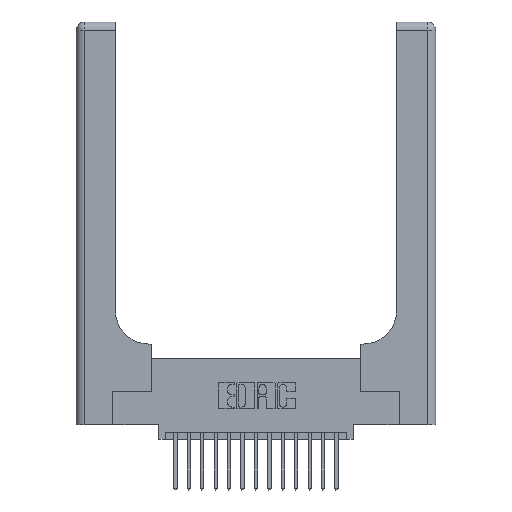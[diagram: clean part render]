
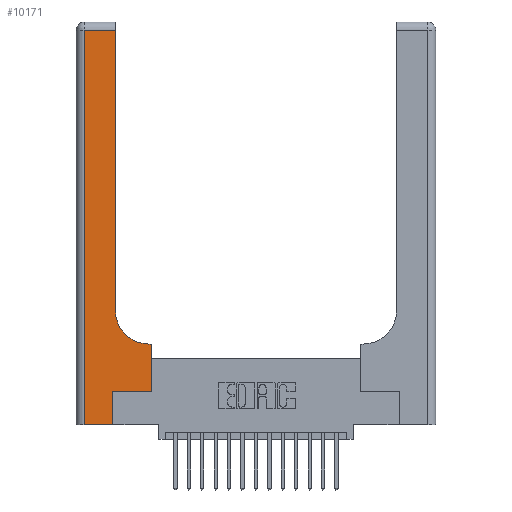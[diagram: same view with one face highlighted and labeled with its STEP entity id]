
A CAD part, top view. The second image highlights one B-rep face of the part: STEP entity #10171.
In plain terms, the highlighted planar face has unit normal (0, 0, 1).
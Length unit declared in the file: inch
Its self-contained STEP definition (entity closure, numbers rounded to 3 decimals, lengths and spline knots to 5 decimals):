
#387 = CARTESIAN_POINT ( 'NONE',  ( 0.5585, 0.25, 0.37 ) ) ;
#643 = VECTOR ( 'NONE', #1100, 39.37008 ) ;
#818 = VECTOR ( 'NONE', #9234, 39.37008 ) ;
#954 = VECTOR ( 'NONE', #3382, 39.37008 ) ;
#1036 = VERTEX_POINT ( 'NONE', #5434 ) ;
#1100 = DIRECTION ( 'NONE',  ( 0., 1., 0. ) ) ;
#1105 = EDGE_CURVE ( 'NONE', #1036, #17673, #13843, .T. ) ;
#1340 = DIRECTION ( 'NONE',  ( 0., 0., -1. ) ) ;
#1770 = CARTESIAN_POINT ( 'NONE',  ( 0., 0., 0.37 ) ) ;
#1915 = CARTESIAN_POINT ( 'NONE',  ( 0.5415, 0.6, 0.37 ) ) ;
#2527 = VECTOR ( 'NONE', #12479, 39.37008 ) ;
#2695 = VERTEX_POINT ( 'NONE', #387 ) ;
#3214 = DIRECTION ( 'NONE',  ( 0., -1., 0. ) ) ;
#3382 = DIRECTION ( 'NONE',  ( 0., 1., 0. ) ) ;
#3685 = ORIENTED_EDGE ( 'NONE', *, *, #6697, .T. ) ;
#3726 = VECTOR ( 'NONE', #6259, 39.37008 ) ;
#3788 = CARTESIAN_POINT ( 'NONE',  ( 0.06, 3., 0.37 ) ) ;
#3835 = VERTEX_POINT ( 'NONE', #15019 ) ;
#3852 = CARTESIAN_POINT ( 'NONE',  ( 0., 3., 0.37 ) ) ;
#5359 = LINE ( 'NONE', #7733, #818 ) ;
#5396 = DIRECTION ( 'NONE',  ( 0., 0., -1. ) ) ;
#5434 = CARTESIAN_POINT ( 'NONE',  ( 0.06, 2.94, 0.37 ) ) ;
#5608 = EDGE_CURVE ( 'NONE', #17673, #18857, #8044, .T. ) ;
#5640 = LINE ( 'NONE', #18066, #16146 ) ;
#5921 = CARTESIAN_POINT ( 'NONE',  ( 0.269, 0., 0.37 ) ) ;
#6138 = ORIENTED_EDGE ( 'NONE', *, *, #1105, .T. ) ;
#6259 = DIRECTION ( 'NONE',  ( 0., 1., 0. ) ) ;
#6562 = LINE ( 'NONE', #18407, #2527 ) ;
#6697 = EDGE_CURVE ( 'NONE', #3835, #1036, #5640, .T. ) ;
#6767 = EDGE_CURVE ( 'NONE', #13712, #3835, #11720, .T. ) ;
#7733 = CARTESIAN_POINT ( 'NONE',  ( 0.2915, 0.6, 0.37 ) ) ;
#7912 = EDGE_CURVE ( 'NONE', #9770, #16740, #5359, .T. ) ;
#8044 = LINE ( 'NONE', #1770, #11524 ) ;
#8713 = LINE ( 'NONE', #19083, #643 ) ;
#8943 = ORIENTED_EDGE ( 'NONE', *, *, #15463, .T. ) ;
#9002 = AXIS2_PLACEMENT_3D ( 'NONE', #10399, #1340, #11905 ) ;
#9234 = DIRECTION ( 'NONE',  ( -1., 0., 0. ) ) ;
#9306 = EDGE_CURVE ( 'NONE', #16740, #13712, #13222, .T. ) ;
#9541 = VERTEX_POINT ( 'NONE', #12407 ) ;
#9770 = VERTEX_POINT ( 'NONE', #17536 ) ;
#10006 = AXIS2_PLACEMENT_3D ( 'NONE', #3852, #5396, #15834 ) ;
#10171 = ADVANCED_FACE ( 'NONE', ( #13188 ), #12836, .F. ) ;
#10252 = ORIENTED_EDGE ( 'NONE', *, *, #9306, .T. ) ;
#10399 = CARTESIAN_POINT ( 'NONE',  ( 0.5415, 0.85, 0.37 ) ) ;
#11524 = VECTOR ( 'NONE', #12252, 39.37008 ) ;
#11720 = LINE ( 'NONE', #12271, #3726 ) ;
#11905 = DIRECTION ( 'NONE',  ( 1., 0., 0. ) ) ;
#12146 = DIRECTION ( 'NONE',  ( -1., 0., 0. ) ) ;
#12252 = DIRECTION ( 'NONE',  ( 1., 0., 0. ) ) ;
#12271 = CARTESIAN_POINT ( 'NONE',  ( 0.2915, 3., 0.37 ) ) ;
#12335 = EDGE_CURVE ( 'NONE', #2695, #9770, #8713, .T. ) ;
#12381 = CARTESIAN_POINT ( 'NONE',  ( 0.269, 0., 0.37 ) ) ;
#12407 = CARTESIAN_POINT ( 'NONE',  ( 0.269, 0.25, 0.37 ) ) ;
#12479 = DIRECTION ( 'NONE',  ( 1., 0., 0. ) ) ;
#12500 = LINE ( 'NONE', #12381, #954 ) ;
#12547 = ORIENTED_EDGE ( 'NONE', *, *, #12335, .T. ) ;
#12701 = EDGE_CURVE ( 'NONE', #9541, #2695, #6562, .T. ) ;
#12804 = EDGE_LOOP ( 'NONE', ( #16137, #3685, #6138, #15274, #8943, #13238, #12547, #15519, #10252 ) ) ;
#12836 = PLANE ( 'NONE',  #10006 ) ;
#13188 = FACE_OUTER_BOUND ( 'NONE', #12804, .T. ) ;
#13222 = CIRCLE ( 'NONE', #9002, 0.25 ) ;
#13238 = ORIENTED_EDGE ( 'NONE', *, *, #12701, .T. ) ;
#13712 = VERTEX_POINT ( 'NONE', #16549 ) ;
#13843 = LINE ( 'NONE', #3788, #16872 ) ;
#15019 = CARTESIAN_POINT ( 'NONE',  ( 0.2915, 2.94, 0.37 ) ) ;
#15274 = ORIENTED_EDGE ( 'NONE', *, *, #5608, .T. ) ;
#15463 = EDGE_CURVE ( 'NONE', #18857, #9541, #12500, .T. ) ;
#15519 = ORIENTED_EDGE ( 'NONE', *, *, #7912, .T. ) ;
#15834 = DIRECTION ( 'NONE',  ( -1., 0., 0. ) ) ;
#16072 = CARTESIAN_POINT ( 'NONE',  ( 0.06, 0., 0.37 ) ) ;
#16137 = ORIENTED_EDGE ( 'NONE', *, *, #6767, .T. ) ;
#16146 = VECTOR ( 'NONE', #12146, 39.37008 ) ;
#16549 = CARTESIAN_POINT ( 'NONE',  ( 0.2915, 0.85, 0.37 ) ) ;
#16740 = VERTEX_POINT ( 'NONE', #1915 ) ;
#16872 = VECTOR ( 'NONE', #3214, 39.37008 ) ;
#17536 = CARTESIAN_POINT ( 'NONE',  ( 0.5585, 0.6, 0.37 ) ) ;
#17673 = VERTEX_POINT ( 'NONE', #16072 ) ;
#18066 = CARTESIAN_POINT ( 'NONE',  ( 0., 2.94, 0.37 ) ) ;
#18407 = CARTESIAN_POINT ( 'NONE',  ( 0.269, 0.25, 0.37 ) ) ;
#18857 = VERTEX_POINT ( 'NONE', #5921 ) ;
#19083 = CARTESIAN_POINT ( 'NONE',  ( 0.5585, 0.25, 0.37 ) ) ;
